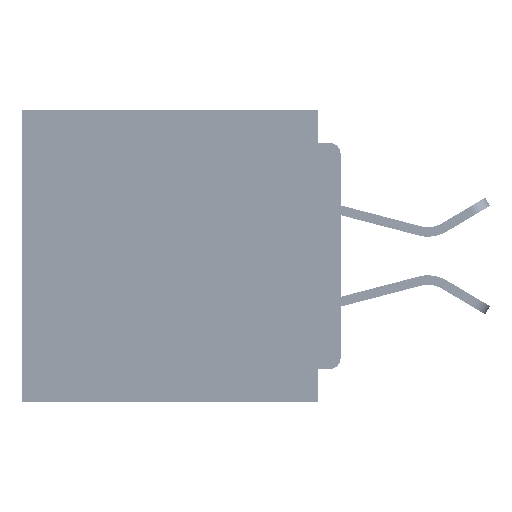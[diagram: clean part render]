
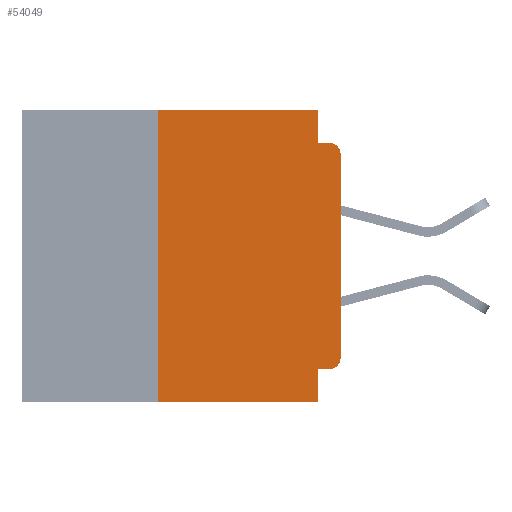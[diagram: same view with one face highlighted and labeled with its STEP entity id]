
A CAD part, left-side view. The second image highlights one B-rep face of the part: STEP entity #54049.
In plain terms, the highlighted planar face has unit normal (-1, 0, 0).
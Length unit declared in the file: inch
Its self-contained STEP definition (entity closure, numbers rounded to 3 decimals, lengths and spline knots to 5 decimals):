
#350 = EDGE_CURVE ( 'NONE', #26603, #1257, #43544, .T. ) ;
#873 = ORIENTED_EDGE ( 'NONE', *, *, #44428, .T. ) ;
#1257 = VERTEX_POINT ( 'NONE', #27755 ) ;
#3711 = CARTESIAN_POINT ( 'NONE',  ( 0., 0.015, -0.34 ) ) ;
#3734 = DIRECTION ( 'NONE',  ( 0., 0., -1. ) ) ;
#4815 = LINE ( 'NONE', #15779, #16623 ) ;
#5310 = DIRECTION ( 'NONE',  ( 0., -1., 0. ) ) ;
#7015 = EDGE_CURVE ( 'NONE', #53428, #37681, #24609, .T. ) ;
#7475 = VECTOR ( 'NONE', #58481, 39.37008 ) ;
#8592 = CARTESIAN_POINT ( 'NONE',  ( 0., 0.437, 0. ) ) ;
#8817 = DIRECTION ( 'NONE',  ( 0., 0., -1. ) ) ;
#9028 = LINE ( 'NONE', #33661, #61656 ) ;
#10072 = CARTESIAN_POINT ( 'NONE',  ( 0., 0.031, 0. ) ) ;
#10656 = CARTESIAN_POINT ( 'NONE',  ( 0., 0.25, -0.4 ) ) ;
#12030 = CARTESIAN_POINT ( 'NONE',  ( 0., 0., -0.045 ) ) ;
#12059 = ORIENTED_EDGE ( 'NONE', *, *, #12061, .T. ) ;
#12061 = EDGE_CURVE ( 'NONE', #62471, #30865, #28007, .T. ) ;
#12680 = CARTESIAN_POINT ( 'NONE',  ( 0., 0.031, -0.045 ) ) ;
#12781 = CARTESIAN_POINT ( 'NONE',  ( 0., 0.25, -0.4 ) ) ;
#14557 = ORIENTED_EDGE ( 'NONE', *, *, #55411, .F. ) ;
#15779 = CARTESIAN_POINT ( 'NONE',  ( 0., 0., 0. ) ) ;
#16623 = VECTOR ( 'NONE', #50426, 39.37008 ) ;
#17176 = VERTEX_POINT ( 'NONE', #12680 ) ;
#17334 = ORIENTED_EDGE ( 'NONE', *, *, #64228, .F. ) ;
#17829 = CARTESIAN_POINT ( 'NONE',  ( 0., 0.031, -0.4 ) ) ;
#18088 = AXIS2_PLACEMENT_3D ( 'NONE', #3711, #38643, #8817 ) ;
#20265 = CARTESIAN_POINT ( 'NONE',  ( 0., 0.437, -0.4 ) ) ;
#20434 = LINE ( 'NONE', #62445, #48333 ) ;
#20549 = ORIENTED_EDGE ( 'NONE', *, *, #7015, .F. ) ;
#20824 = LINE ( 'NONE', #28948, #7475 ) ;
#21491 = ORIENTED_EDGE ( 'NONE', *, *, #350, .T. ) ;
#21859 = DIRECTION ( 'NONE',  ( 0., -1., 0. ) ) ;
#21897 = EDGE_CURVE ( 'NONE', #53428, #54776, #48963, .T. ) ;
#21933 = VECTOR ( 'NONE', #21859, 39.37008 ) ;
#22077 = VECTOR ( 'NONE', #43390, 39.37008 ) ;
#22517 = CARTESIAN_POINT ( 'NONE',  ( 0., 0.031, -0.355 ) ) ;
#23719 = DIRECTION ( 'NONE',  ( 0., 0., -1. ) ) ;
#23795 = DIRECTION ( 'NONE',  ( -1., 0., 0. ) ) ;
#23806 = CARTESIAN_POINT ( 'NONE',  ( 0., 0.015, -0.06 ) ) ;
#24235 = EDGE_CURVE ( 'NONE', #37127, #54776, #9028, .T. ) ;
#24609 = LINE ( 'NONE', #10656, #36146 ) ;
#25229 = AXIS2_PLACEMENT_3D ( 'NONE', #23806, #23795, #23719 ) ;
#26409 = DIRECTION ( 'NONE',  ( 1., 0., 0. ) ) ;
#26603 = VERTEX_POINT ( 'NONE', #49485 ) ;
#27755 = CARTESIAN_POINT ( 'NONE',  ( 0., 0.015, -0.045 ) ) ;
#28007 = CIRCLE ( 'NONE', #18088, 0.015 ) ;
#28948 = CARTESIAN_POINT ( 'NONE',  ( 0., 0.031, 0. ) ) ;
#30865 = VERTEX_POINT ( 'NONE', #39320 ) ;
#31536 = CARTESIAN_POINT ( 'NONE',  ( 0., 0.25, 0. ) ) ;
#31594 = ORIENTED_EDGE ( 'NONE', *, *, #43586, .F. ) ;
#32382 = ORIENTED_EDGE ( 'NONE', *, *, #21897, .T. ) ;
#32935 = DIRECTION ( 'NONE',  ( 0., 1., 0. ) ) ;
#33661 = CARTESIAN_POINT ( 'NONE',  ( 0., 0.031, -0.4 ) ) ;
#35756 = VECTOR ( 'NONE', #5310, 39.37008 ) ;
#35998 = ORIENTED_EDGE ( 'NONE', *, *, #55821, .F. ) ;
#36146 = VECTOR ( 'NONE', #40849, 39.37008 ) ;
#36773 = EDGE_LOOP ( 'NONE', ( #873, #21491, #35998, #31594, #17334, #20549, #32382, #61390, #14557, #12059 ) ) ;
#37127 = VERTEX_POINT ( 'NONE', #22517 ) ;
#37681 = VERTEX_POINT ( 'NONE', #31536 ) ;
#38643 = DIRECTION ( 'NONE',  ( -1., 0., 0. ) ) ;
#39320 = CARTESIAN_POINT ( 'NONE',  ( 0., 0., -0.34 ) ) ;
#40849 = DIRECTION ( 'NONE',  ( 0., 0., 1. ) ) ;
#41126 = CARTESIAN_POINT ( 'NONE',  ( 0., 0.437, 0. ) ) ;
#41560 = FACE_OUTER_BOUND ( 'NONE', #36773, .T. ) ;
#43390 = DIRECTION ( 'NONE',  ( 0., -1., 0. ) ) ;
#43544 = CIRCLE ( 'NONE', #25229, 0.015 ) ;
#43586 = EDGE_CURVE ( 'NONE', #58004, #17176, #20824, .T. ) ;
#44428 = EDGE_CURVE ( 'NONE', #30865, #26603, #4815, .T. ) ;
#48333 = VECTOR ( 'NONE', #32935, 39.37008 ) ;
#48963 = LINE ( 'NONE', #20265, #35756 ) ;
#49485 = CARTESIAN_POINT ( 'NONE',  ( 0., 0., -0.06 ) ) ;
#50426 = DIRECTION ( 'NONE',  ( 0., 0., 1. ) ) ;
#53428 = VERTEX_POINT ( 'NONE', #12781 ) ;
#54049 = ADVANCED_FACE ( 'NONE', ( #41560 ), #55968, .F. ) ;
#54776 = VERTEX_POINT ( 'NONE', #17829 ) ;
#55411 = EDGE_CURVE ( 'NONE', #62471, #37127, #20434, .T. ) ;
#55821 = EDGE_CURVE ( 'NONE', #17176, #1257, #61277, .T. ) ;
#55968 = PLANE ( 'NONE',  #60898 ) ;
#58004 = VERTEX_POINT ( 'NONE', #10072 ) ;
#58481 = DIRECTION ( 'NONE',  ( 0., 0., -1. ) ) ;
#59892 = LINE ( 'NONE', #8592, #22077 ) ;
#60878 = DIRECTION ( 'NONE',  ( 0., 0., -1. ) ) ;
#60898 = AXIS2_PLACEMENT_3D ( 'NONE', #41126, #26409, #60878 ) ;
#61277 = LINE ( 'NONE', #12030, #21933 ) ;
#61390 = ORIENTED_EDGE ( 'NONE', *, *, #24235, .F. ) ;
#61656 = VECTOR ( 'NONE', #3734, 39.37008 ) ;
#62445 = CARTESIAN_POINT ( 'NONE',  ( 0., 0., -0.355 ) ) ;
#62471 = VERTEX_POINT ( 'NONE', #63538 ) ;
#63538 = CARTESIAN_POINT ( 'NONE',  ( 0., 0.015, -0.355 ) ) ;
#64228 = EDGE_CURVE ( 'NONE', #37681, #58004, #59892, .T. ) ;
